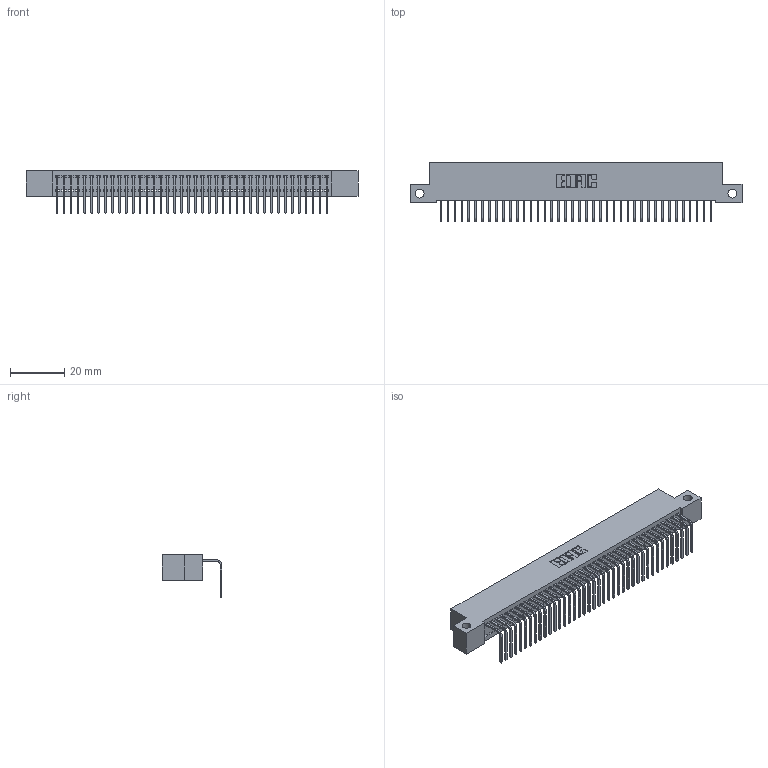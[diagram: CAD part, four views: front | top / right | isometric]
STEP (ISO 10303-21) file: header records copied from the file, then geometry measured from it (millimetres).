
FILE_DESCRIPTION (( 'STEP AP203' ), '1' );
FILE_NAME ('342-040-558-112.STEP', '2019-10-02T17:03:30', ( '' ), ( '' ), 'SwSTEP 2.0', 'SolidWorks 2016', '' );
FILE_SCHEMA (( 'CONFIG_CONTROL_DESIGN' ));
Length unit declared in the file: inch
Products named in the file (3): 345-292-001_558 Tail - 2; 342-040-558-112; 342 Part_Side Mount
Assembly tree (41 placements, depth 2):
  342-040-558-112
    342 Part_Side Mount
    345-292-001_558 Tail - 2  x40
Bounding box: 121.92 x 21.91 x 15.62 mm (x, y, z)
Volume: 10741.9 mm3; surface area: 16330.5 mm2
Topology: 41 solids, 41 shells, 2510 faces, 7579 edges, 4998 vertices
Faces by surface type: plane 1826, cylinder 684
Entity records: 24667 total; most frequent: CARTESIAN_POINT 4262, ORIENTED_EDGE 4238, DIRECTION 3599, EDGE_CURVE 2119, VECTOR 1991, LINE 1991, VERTEX_POINT 1410, AXIS2_PLACEMENT_3D 804
